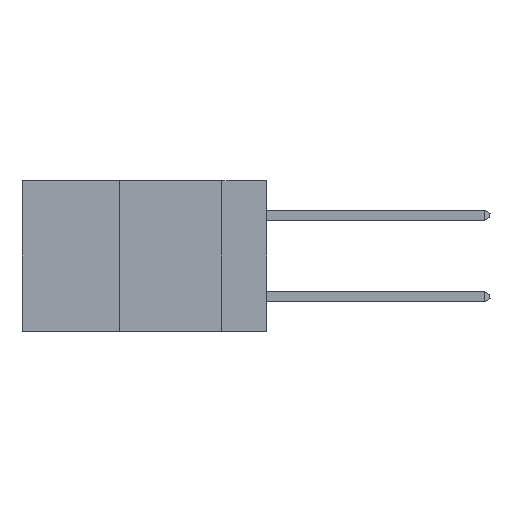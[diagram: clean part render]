
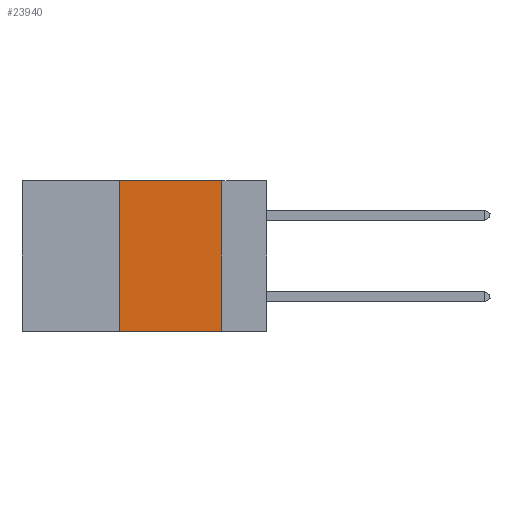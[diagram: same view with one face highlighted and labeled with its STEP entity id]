
A CAD part, left-side view. The second image highlights one B-rep face of the part: STEP entity #23940.
In plain terms, the highlighted planar face has unit normal (-1, 0, 0).
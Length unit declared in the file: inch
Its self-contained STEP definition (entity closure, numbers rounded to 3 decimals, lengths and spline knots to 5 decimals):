
#2074 = CARTESIAN_POINT ( 'NONE',  ( 0., 0.6, 0. ) ) ;
#2811 = DIRECTION ( 'NONE',  ( 0., -1., 0. ) ) ;
#2950 = VERTEX_POINT ( 'NONE', #18473 ) ;
#4548 = CARTESIAN_POINT ( 'NONE',  ( 0., 0.6, 0. ) ) ;
#6407 = PLANE ( 'NONE',  #12084 ) ;
#6481 = DIRECTION ( 'NONE',  ( 0., 0., -1. ) ) ;
#6647 = EDGE_CURVE ( 'NONE', #16546, #2950, #22520, .T. ) ;
#6985 = CARTESIAN_POINT ( 'NONE',  ( 0., 0.36, 0. ) ) ;
#7564 = LINE ( 'NONE', #15101, #12034 ) ;
#8072 = EDGE_LOOP ( 'NONE', ( #17091, #17693, #22624, #13807 ) ) ;
#8264 = EDGE_CURVE ( 'NONE', #19990, #9895, #10952, .T. ) ;
#9895 = VERTEX_POINT ( 'NONE', #13956 ) ;
#10952 = LINE ( 'NONE', #2074, #16028 ) ;
#12034 = VECTOR ( 'NONE', #18894, 39.37008 ) ;
#12084 = AXIS2_PLACEMENT_3D ( 'NONE', #4548, #17847, #6481 ) ;
#12091 = CARTESIAN_POINT ( 'NONE',  ( 0., 0.11, 0. ) ) ;
#13807 = ORIENTED_EDGE ( 'NONE', *, *, #6647, .T. ) ;
#13956 = CARTESIAN_POINT ( 'NONE',  ( 0., 0.11, 0. ) ) ;
#15101 = CARTESIAN_POINT ( 'NONE',  ( 0., 0.36, 0. ) ) ;
#15460 = DIRECTION ( 'NONE',  ( 0., -1., 0. ) ) ;
#16028 = VECTOR ( 'NONE', #15460, 39.37008 ) ;
#16546 = VERTEX_POINT ( 'NONE', #19381 ) ;
#17091 = ORIENTED_EDGE ( 'NONE', *, *, #17755, .F. ) ;
#17600 = VECTOR ( 'NONE', #2811, 39.37008 ) ;
#17693 = ORIENTED_EDGE ( 'NONE', *, *, #8264, .F. ) ;
#17755 = EDGE_CURVE ( 'NONE', #9895, #2950, #23890, .T. ) ;
#17847 = DIRECTION ( 'NONE',  ( 1., 0., 0. ) ) ;
#18473 = CARTESIAN_POINT ( 'NONE',  ( 0., 0.11, -0.37 ) ) ;
#18894 = DIRECTION ( 'NONE',  ( 0., 0., 1. ) ) ;
#19381 = CARTESIAN_POINT ( 'NONE',  ( 0., 0.36, -0.37 ) ) ;
#19878 = CARTESIAN_POINT ( 'NONE',  ( 0., 0.6, -0.37 ) ) ;
#19990 = VERTEX_POINT ( 'NONE', #6985 ) ;
#21815 = EDGE_CURVE ( 'NONE', #16546, #19990, #7564, .T. ) ;
#21909 = FACE_OUTER_BOUND ( 'NONE', #8072, .T. ) ;
#22520 = LINE ( 'NONE', #19878, #17600 ) ;
#22624 = ORIENTED_EDGE ( 'NONE', *, *, #21815, .F. ) ;
#23332 = DIRECTION ( 'NONE',  ( 0., 0., -1. ) ) ;
#23336 = VECTOR ( 'NONE', #23332, 39.37008 ) ;
#23890 = LINE ( 'NONE', #12091, #23336 ) ;
#23940 = ADVANCED_FACE ( 'NONE', ( #21909 ), #6407, .F. ) ;
